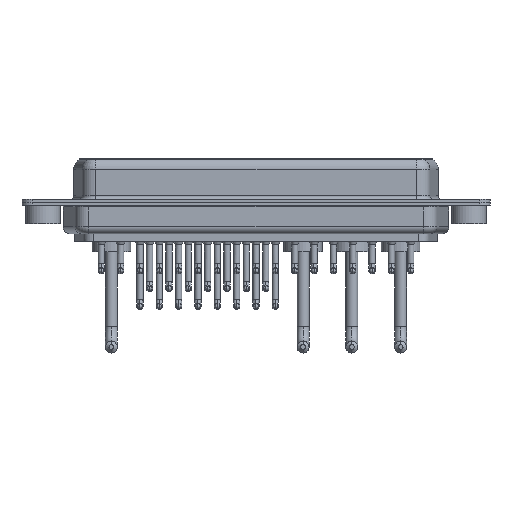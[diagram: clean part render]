
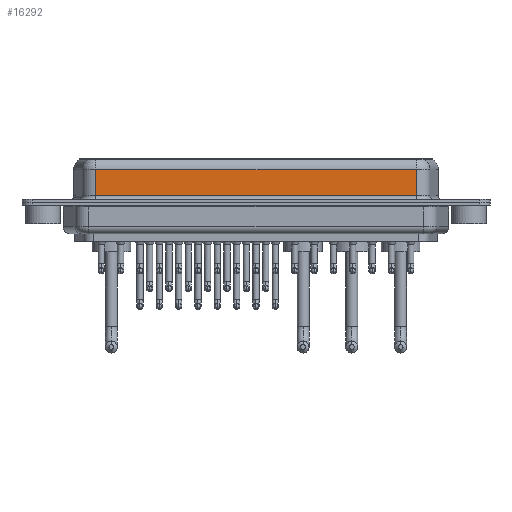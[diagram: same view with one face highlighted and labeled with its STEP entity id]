
A CAD part, front view. The second image highlights one B-rep face of the part: STEP entity #16292.
In plain terms, the highlighted planar face has unit normal (0, -1, 0).
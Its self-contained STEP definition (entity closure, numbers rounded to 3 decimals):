
#522 = EDGE_CURVE ( 'NONE', #7137, #3176, #26402, .T. ) ;
#876 = EDGE_CURVE ( 'NONE', #20781, #15314, #25199, .T. ) ;
#1250 = ORIENTED_EDGE ( 'NONE', *, *, #876, .T. ) ;
#1877 = VECTOR ( 'NONE', #5191, 1000. ) ;
#2298 = AXIS2_PLACEMENT_3D ( 'NONE', #21731, #12392, #8091 ) ;
#3176 = VERTEX_POINT ( 'NONE', #14469 ) ;
#3512 = PLANE ( 'NONE',  #2298 ) ;
#3756 = CARTESIAN_POINT ( 'NONE',  ( 53.41, -5.375, 0.9 ) ) ;
#4057 = VECTOR ( 'NONE', #16310, 1000. ) ;
#5191 = DIRECTION ( 'NONE',  ( -1., 0., 0. ) ) ;
#5386 = ORIENTED_EDGE ( 'NONE', *, *, #12112, .F. ) ;
#7137 = VERTEX_POINT ( 'NONE', #9518 ) ;
#8091 = DIRECTION ( 'NONE',  ( 0., 0., 1. ) ) ;
#9495 = CARTESIAN_POINT ( 'NONE',  ( 7.59, -5.375, 6.4 ) ) ;
#9499 = LINE ( 'NONE', #20351, #16514 ) ;
#9518 = CARTESIAN_POINT ( 'NONE',  ( 7.59, -5.375, 0.9 ) ) ;
#9735 = VECTOR ( 'NONE', #25961, 1000. ) ;
#11292 = CARTESIAN_POINT ( 'NONE',  ( 53.41, -5.375, 4.65 ) ) ;
#12112 = EDGE_CURVE ( 'NONE', #20781, #3176, #9499, .T. ) ;
#12392 = DIRECTION ( 'NONE',  ( 0., 1., 0. ) ) ;
#14469 = CARTESIAN_POINT ( 'NONE',  ( 53.41, -5.375, 0.9 ) ) ;
#15314 = VERTEX_POINT ( 'NONE', #25947 ) ;
#15481 = EDGE_LOOP ( 'NONE', ( #5386, #1250, #18146, #28325 ) ) ;
#16032 = LINE ( 'NONE', #9495, #4057 ) ;
#16292 = ADVANCED_FACE ( 'NONE', ( #28114 ), #3512, .F. ) ;
#16310 = DIRECTION ( 'NONE',  ( 0., 0., -1. ) ) ;
#16514 = VECTOR ( 'NONE', #25217, 1000. ) ;
#18146 = ORIENTED_EDGE ( 'NONE', *, *, #27903, .T. ) ;
#20351 = CARTESIAN_POINT ( 'NONE',  ( 53.41, -5.375, 6.4 ) ) ;
#20781 = VERTEX_POINT ( 'NONE', #11292 ) ;
#21731 = CARTESIAN_POINT ( 'NONE',  ( 53.41, -5.375, 6.4 ) ) ;
#23126 = CARTESIAN_POINT ( 'NONE',  ( 53.41, -5.375, 4.65 ) ) ;
#25199 = LINE ( 'NONE', #23126, #1877 ) ;
#25217 = DIRECTION ( 'NONE',  ( 0., 0., -1. ) ) ;
#25947 = CARTESIAN_POINT ( 'NONE',  ( 7.59, -5.375, 4.65 ) ) ;
#25961 = DIRECTION ( 'NONE',  ( 1., 0., 0. ) ) ;
#26402 = LINE ( 'NONE', #3756, #9735 ) ;
#27903 = EDGE_CURVE ( 'NONE', #15314, #7137, #16032, .T. ) ;
#28114 = FACE_OUTER_BOUND ( 'NONE', #15481, .T. ) ;
#28325 = ORIENTED_EDGE ( 'NONE', *, *, #522, .T. ) ;
